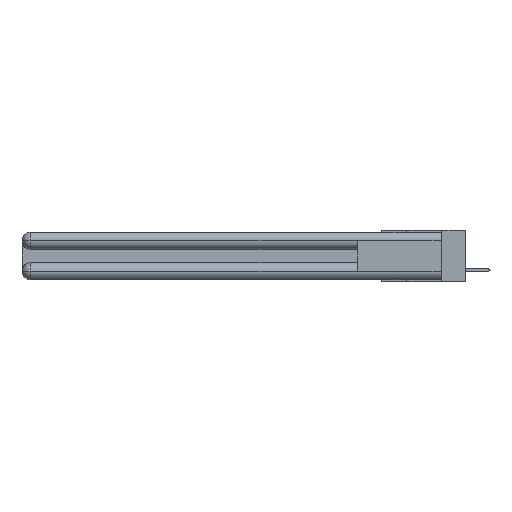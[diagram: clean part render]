
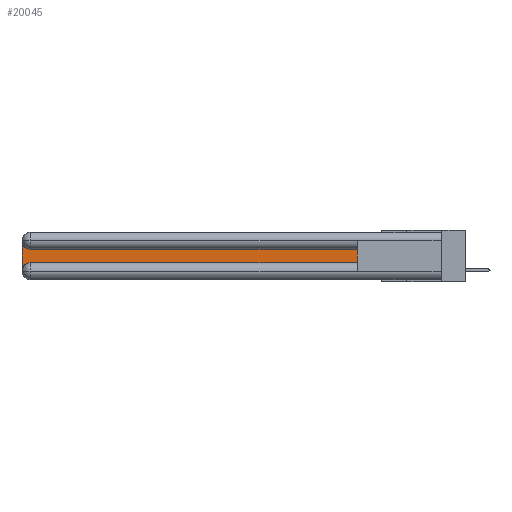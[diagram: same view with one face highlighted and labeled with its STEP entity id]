
A CAD part, left-side view. The second image highlights one B-rep face of the part: STEP entity #20045.
In plain terms, the highlighted planar face has unit normal (-1, 0, 0).
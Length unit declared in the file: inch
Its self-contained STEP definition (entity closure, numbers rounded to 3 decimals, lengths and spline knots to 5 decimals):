
#5 = DIRECTION ( 'NONE',  ( 0., 1., 0. ) ) ;
#538 = LINE ( 'NONE', #18210, #20633 ) ;
#1083 = VERTEX_POINT ( 'NONE', #14168 ) ;
#1239 = VECTOR ( 'NONE', #10978, 39.37008 ) ;
#1595 = ORIENTED_EDGE ( 'NONE', *, *, #9830, .T. ) ;
#1663 = ORIENTED_EDGE ( 'NONE', *, *, #11723, .T. ) ;
#2269 = CARTESIAN_POINT ( 'NONE',  ( 0.075, 2.94, -0.2775 ) ) ;
#2902 = AXIS2_PLACEMENT_3D ( 'NONE', #2269, #30355, #23136 ) ;
#3038 = VERTEX_POINT ( 'NONE', #20381 ) ;
#3416 = DIRECTION ( 'NONE',  ( 1., 0., 0. ) ) ;
#4770 = CARTESIAN_POINT ( 'NONE',  ( 0.075, 0.6, -0.2175 ) ) ;
#5874 = VECTOR ( 'NONE', #5, 39.37008 ) ;
#7861 = DIRECTION ( 'NONE',  ( 0., 0., -1. ) ) ;
#8359 = AXIS2_PLACEMENT_3D ( 'NONE', #15252, #3416, #19964 ) ;
#8402 = EDGE_CURVE ( 'NONE', #22429, #1083, #16845, .T. ) ;
#8961 = ORIENTED_EDGE ( 'NONE', *, *, #27080, .T. ) ;
#8976 = CARTESIAN_POINT ( 'NONE',  ( 0.075, 0.6, -0.1225 ) ) ;
#9752 = AXIS2_PLACEMENT_3D ( 'NONE', #26865, #17595, #7861 ) ;
#9830 = EDGE_CURVE ( 'NONE', #1083, #3038, #19288, .T. ) ;
#10170 = ORIENTED_EDGE ( 'NONE', *, *, #18455, .T. ) ;
#10978 = DIRECTION ( 'NONE',  ( 0., 0., 1. ) ) ;
#11723 = EDGE_CURVE ( 'NONE', #22213, #22429, #26146, .T. ) ;
#13985 = EDGE_CURVE ( 'NONE', #3038, #30160, #16790, .T. ) ;
#14041 = ORIENTED_EDGE ( 'NONE', *, *, #13985, .T. ) ;
#14168 = CARTESIAN_POINT ( 'NONE',  ( 0.075, 2.94, -0.1225 ) ) ;
#15252 = CARTESIAN_POINT ( 'NONE',  ( 0.075, 3., -0.1225 ) ) ;
#15257 = VERTEX_POINT ( 'NONE', #26058 ) ;
#16790 = LINE ( 'NONE', #19823, #20850 ) ;
#16845 = LINE ( 'NONE', #20675, #5874 ) ;
#17595 = DIRECTION ( 'NONE',  ( 1., 0., 0. ) ) ;
#18210 = CARTESIAN_POINT ( 'NONE',  ( 0.075, 0.6, -0.2175 ) ) ;
#18455 = EDGE_CURVE ( 'NONE', #30160, #15257, #25300, .T. ) ;
#18633 = ORIENTED_EDGE ( 'NONE', *, *, #8402, .T. ) ;
#18796 = EDGE_LOOP ( 'NONE', ( #18633, #1595, #14041, #10170, #8961, #1663 ) ) ;
#19288 = CIRCLE ( 'NONE', #9752, 0.06 ) ;
#19716 = CARTESIAN_POINT ( 'NONE',  ( 0.075, 0.6, -0.2175 ) ) ;
#19823 = CARTESIAN_POINT ( 'NONE',  ( 0.075, 3., -0.2175 ) ) ;
#19964 = DIRECTION ( 'NONE',  ( 0., 0., -1. ) ) ;
#20045 = ADVANCED_FACE ( 'NONE', ( #21447 ), #26771, .F. ) ;
#20381 = CARTESIAN_POINT ( 'NONE',  ( 0.075, 3., -0.0625 ) ) ;
#20633 = VECTOR ( 'NONE', #23143, 39.37008 ) ;
#20675 = CARTESIAN_POINT ( 'NONE',  ( 0.075, 0.6, -0.1225 ) ) ;
#20850 = VECTOR ( 'NONE', #28816, 39.37008 ) ;
#21447 = FACE_OUTER_BOUND ( 'NONE', #18796, .T. ) ;
#22213 = VERTEX_POINT ( 'NONE', #19716 ) ;
#22429 = VERTEX_POINT ( 'NONE', #8976 ) ;
#23136 = DIRECTION ( 'NONE',  ( 0., 0., -1. ) ) ;
#23143 = DIRECTION ( 'NONE',  ( 0., -1., 0. ) ) ;
#25022 = CARTESIAN_POINT ( 'NONE',  ( 0.075, 3., -0.2775 ) ) ;
#25300 = CIRCLE ( 'NONE', #2902, 0.06 ) ;
#26058 = CARTESIAN_POINT ( 'NONE',  ( 0.075, 2.94, -0.2175 ) ) ;
#26146 = LINE ( 'NONE', #4770, #1239 ) ;
#26771 = PLANE ( 'NONE',  #8359 ) ;
#26865 = CARTESIAN_POINT ( 'NONE',  ( 0.075, 2.94, -0.0625 ) ) ;
#27080 = EDGE_CURVE ( 'NONE', #15257, #22213, #538, .T. ) ;
#28816 = DIRECTION ( 'NONE',  ( 0., 0., -1. ) ) ;
#30160 = VERTEX_POINT ( 'NONE', #25022 ) ;
#30355 = DIRECTION ( 'NONE',  ( 1., 0., 0. ) ) ;
